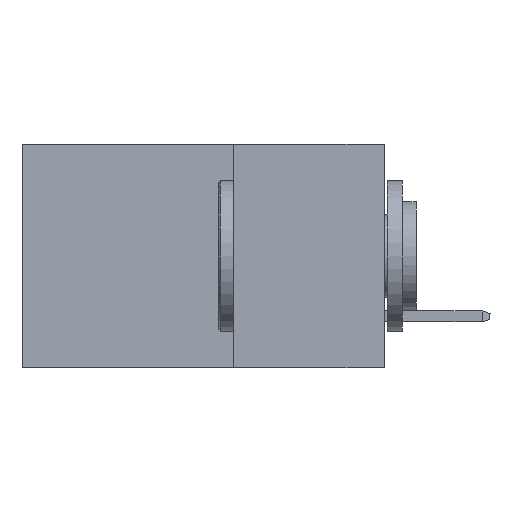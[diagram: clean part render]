
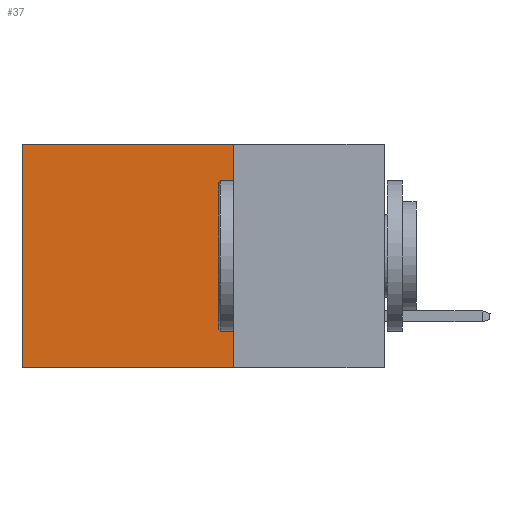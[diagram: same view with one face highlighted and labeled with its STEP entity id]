
A CAD part, left-side view. The second image highlights one B-rep face of the part: STEP entity #37.
In plain terms, the highlighted planar face has unit normal (-1, 0, 0).
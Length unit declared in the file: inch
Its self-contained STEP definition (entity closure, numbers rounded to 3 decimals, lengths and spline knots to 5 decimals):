
#17 = CARTESIAN_POINT ( 'NONE',  ( 0.2615, 0.6, -0.37 ) ) ;
#37 = ADVANCED_FACE ( 'NONE', ( #11077 ), #13831, .F. ) ;
#421 = ORIENTED_EDGE ( 'NONE', *, *, #16087, .F. ) ;
#584 = LINE ( 'NONE', #3062, #8162 ) ;
#1140 = DIRECTION ( 'NONE',  ( 0., 1., 0. ) ) ;
#1144 = VECTOR ( 'NONE', #16328, 39.37008 ) ;
#2046 = CARTESIAN_POINT ( 'NONE',  ( 0.2615, 0.25, 0. ) ) ;
#2268 = ORIENTED_EDGE ( 'NONE', *, *, #3268, .F. ) ;
#2448 = CARTESIAN_POINT ( 'NONE',  ( 0.2615, 0.25, -0.37 ) ) ;
#2655 = EDGE_CURVE ( 'NONE', #7097, #5476, #584, .T. ) ;
#3062 = CARTESIAN_POINT ( 'NONE',  ( 0.2615, 0.6, -0.37 ) ) ;
#3181 = VERTEX_POINT ( 'NONE', #4772 ) ;
#3268 = EDGE_CURVE ( 'NONE', #3181, #13499, #7694, .T. ) ;
#3608 = EDGE_LOOP ( 'NONE', ( #9760, #421, #2268, #16074 ) ) ;
#4772 = CARTESIAN_POINT ( 'NONE',  ( 0.2615, 0.25, 0. ) ) ;
#5274 = CARTESIAN_POINT ( 'NONE',  ( 0.2615, 0.25, -0.37 ) ) ;
#5476 = VERTEX_POINT ( 'NONE', #17 ) ;
#5612 = EDGE_CURVE ( 'NONE', #3181, #7097, #15708, .T. ) ;
#6818 = VECTOR ( 'NONE', #1140, 39.37008 ) ;
#6954 = LINE ( 'NONE', #2448, #6818 ) ;
#7097 = VERTEX_POINT ( 'NONE', #13092 ) ;
#7608 = DIRECTION ( 'NONE',  ( 0., 1., 0. ) ) ;
#7694 = LINE ( 'NONE', #12075, #1144 ) ;
#8064 = AXIS2_PLACEMENT_3D ( 'NONE', #5274, #8355, #9649 ) ;
#8162 = VECTOR ( 'NONE', #17096, 39.37008 ) ;
#8355 = DIRECTION ( 'NONE',  ( 1., 0., 0. ) ) ;
#9649 = DIRECTION ( 'NONE',  ( 0., 0., -1. ) ) ;
#9760 = ORIENTED_EDGE ( 'NONE', *, *, #2655, .T. ) ;
#11077 = FACE_OUTER_BOUND ( 'NONE', #3608, .T. ) ;
#12075 = CARTESIAN_POINT ( 'NONE',  ( 0.2615, 0.25, -0.37 ) ) ;
#13092 = CARTESIAN_POINT ( 'NONE',  ( 0.2615, 0.6, 0. ) ) ;
#13499 = VERTEX_POINT ( 'NONE', #14352 ) ;
#13723 = VECTOR ( 'NONE', #7608, 39.37008 ) ;
#13831 = PLANE ( 'NONE',  #8064 ) ;
#14352 = CARTESIAN_POINT ( 'NONE',  ( 0.2615, 0.25, -0.37 ) ) ;
#15708 = LINE ( 'NONE', #2046, #13723 ) ;
#16074 = ORIENTED_EDGE ( 'NONE', *, *, #5612, .T. ) ;
#16087 = EDGE_CURVE ( 'NONE', #13499, #5476, #6954, .T. ) ;
#16328 = DIRECTION ( 'NONE',  ( 0., 0., -1. ) ) ;
#17096 = DIRECTION ( 'NONE',  ( 0., 0., -1. ) ) ;
